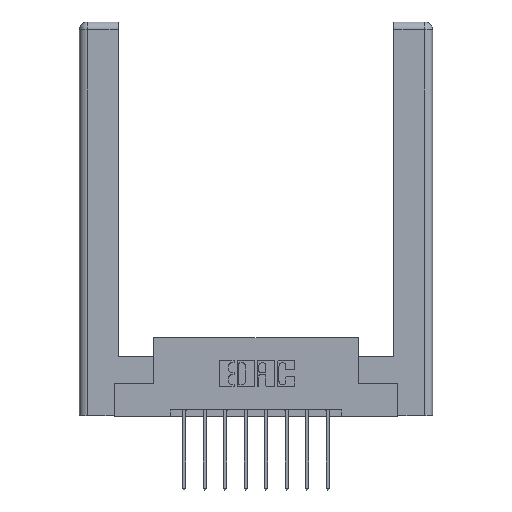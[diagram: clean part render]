
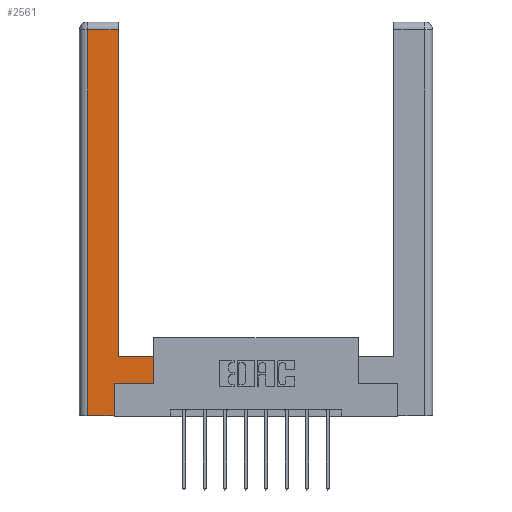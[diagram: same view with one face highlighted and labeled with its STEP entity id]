
A CAD part, top view. The second image highlights one B-rep face of the part: STEP entity #2561.
In plain terms, the highlighted planar face has unit normal (0, 0, 1).
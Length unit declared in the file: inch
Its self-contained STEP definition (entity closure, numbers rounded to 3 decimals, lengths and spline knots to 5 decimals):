
#265 = CARTESIAN_POINT ( 'NONE',  ( 0.565, 0.245, 0. ) ) ;
#473 = DIRECTION ( 'NONE',  ( 0., 1., 0. ) ) ;
#502 = ORIENTED_EDGE ( 'NONE', *, *, #12801, .T. ) ;
#826 = LINE ( 'NONE', #5272, #7708 ) ;
#993 = FACE_OUTER_BOUND ( 'NONE', #12713, .T. ) ;
#1225 = VERTEX_POINT ( 'NONE', #12985 ) ;
#1762 = CARTESIAN_POINT ( 'NONE',  ( 0.265, 0., 0. ) ) ;
#1781 = AXIS2_PLACEMENT_3D ( 'NONE', #12399, #7229, #3084 ) ;
#1860 = VERTEX_POINT ( 'NONE', #265 ) ;
#2061 = DIRECTION ( 'NONE',  ( -1., 0., 0. ) ) ;
#2169 = DIRECTION ( 'NONE',  ( 0., 1., 0. ) ) ;
#2232 = ORIENTED_EDGE ( 'NONE', *, *, #3223, .T. ) ;
#2287 = CARTESIAN_POINT ( 'NONE',  ( 0.295, 0.45, 0. ) ) ;
#2561 = ADVANCED_FACE ( 'NONE', ( #993 ), #8198, .F. ) ;
#3084 = DIRECTION ( 'NONE',  ( -1., 0., 0. ) ) ;
#3111 = ORIENTED_EDGE ( 'NONE', *, *, #3126, .T. ) ;
#3126 = EDGE_CURVE ( 'NONE', #6634, #5068, #7548, .T. ) ;
#3223 = EDGE_CURVE ( 'NONE', #5722, #7697, #12021, .T. ) ;
#3463 = ORIENTED_EDGE ( 'NONE', *, *, #12091, .T. ) ;
#3616 = CARTESIAN_POINT ( 'NONE',  ( 0.265, 0.245, 0. ) ) ;
#3847 = DIRECTION ( 'NONE',  ( 1., 0., 0. ) ) ;
#4170 = VECTOR ( 'NONE', #2061, 39.37008 ) ;
#4361 = LINE ( 'NONE', #1762, #13013 ) ;
#4684 = DIRECTION ( 'NONE',  ( -1., 0., 0. ) ) ;
#4725 = CARTESIAN_POINT ( 'NONE',  ( 0.295, 2.94, 0. ) ) ;
#4796 = CARTESIAN_POINT ( 'NONE',  ( 0.295, 3., 0. ) ) ;
#4869 = ORIENTED_EDGE ( 'NONE', *, *, #9995, .T. ) ;
#5068 = VERTEX_POINT ( 'NONE', #12915 ) ;
#5272 = CARTESIAN_POINT ( 'NONE',  ( 0.265, 0.245, 0. ) ) ;
#5323 = VERTEX_POINT ( 'NONE', #10968 ) ;
#5397 = LINE ( 'NONE', #6750, #6360 ) ;
#5607 = EDGE_CURVE ( 'NONE', #10250, #1860, #5397, .T. ) ;
#5722 = VERTEX_POINT ( 'NONE', #10219 ) ;
#6360 = VECTOR ( 'NONE', #9875, 39.37008 ) ;
#6510 = VECTOR ( 'NONE', #8829, 39.37008 ) ;
#6600 = ORIENTED_EDGE ( 'NONE', *, *, #9137, .T. ) ;
#6634 = VERTEX_POINT ( 'NONE', #4725 ) ;
#6750 = CARTESIAN_POINT ( 'NONE',  ( 0.565, 0.245, 0. ) ) ;
#7179 = CARTESIAN_POINT ( 'NONE',  ( 0.0615, 2.94, 0. ) ) ;
#7229 = DIRECTION ( 'NONE',  ( 0., 0., -1. ) ) ;
#7383 = VECTOR ( 'NONE', #4684, 39.37008 ) ;
#7514 = DIRECTION ( 'NONE',  ( 0., -1., 0. ) ) ;
#7548 = LINE ( 'NONE', #7179, #4170 ) ;
#7697 = VERTEX_POINT ( 'NONE', #2287 ) ;
#7708 = VECTOR ( 'NONE', #2169, 39.37008 ) ;
#7806 = EDGE_CURVE ( 'NONE', #5068, #1225, #10740, .T. ) ;
#7826 = CARTESIAN_POINT ( 'NONE',  ( 0.295, 0.45, 0. ) ) ;
#8198 = PLANE ( 'NONE',  #1781 ) ;
#8448 = VECTOR ( 'NONE', #473, 39.37008 ) ;
#8620 = CARTESIAN_POINT ( 'NONE',  ( 0.565, 0.45, 0. ) ) ;
#8829 = DIRECTION ( 'NONE',  ( 0., 1., 0. ) ) ;
#9137 = EDGE_CURVE ( 'NONE', #1860, #5722, #11955, .T. ) ;
#9617 = ORIENTED_EDGE ( 'NONE', *, *, #5607, .T. ) ;
#9875 = DIRECTION ( 'NONE',  ( 1., 0., 0. ) ) ;
#9995 = EDGE_CURVE ( 'NONE', #7697, #6634, #11940, .T. ) ;
#10219 = CARTESIAN_POINT ( 'NONE',  ( 0.565, 0.45, 0. ) ) ;
#10250 = VERTEX_POINT ( 'NONE', #3616 ) ;
#10438 = CARTESIAN_POINT ( 'NONE',  ( 0.0615, 0., 0. ) ) ;
#10585 = VECTOR ( 'NONE', #7514, 39.37008 ) ;
#10740 = LINE ( 'NONE', #10438, #10585 ) ;
#10968 = CARTESIAN_POINT ( 'NONE',  ( 0.265, 0., 0. ) ) ;
#11884 = ORIENTED_EDGE ( 'NONE', *, *, #7806, .T. ) ;
#11940 = LINE ( 'NONE', #4796, #6510 ) ;
#11955 = LINE ( 'NONE', #8620, #8448 ) ;
#12021 = LINE ( 'NONE', #7826, #7383 ) ;
#12091 = EDGE_CURVE ( 'NONE', #1225, #5323, #4361, .T. ) ;
#12399 = CARTESIAN_POINT ( 'NONE',  ( 0., 0., 0. ) ) ;
#12713 = EDGE_LOOP ( 'NONE', ( #4869, #3111, #11884, #3463, #502, #9617, #6600, #2232 ) ) ;
#12801 = EDGE_CURVE ( 'NONE', #5323, #10250, #826, .T. ) ;
#12915 = CARTESIAN_POINT ( 'NONE',  ( 0.0615, 2.94, 0. ) ) ;
#12985 = CARTESIAN_POINT ( 'NONE',  ( 0.0615, 0., 0. ) ) ;
#13013 = VECTOR ( 'NONE', #3847, 39.37008 ) ;
